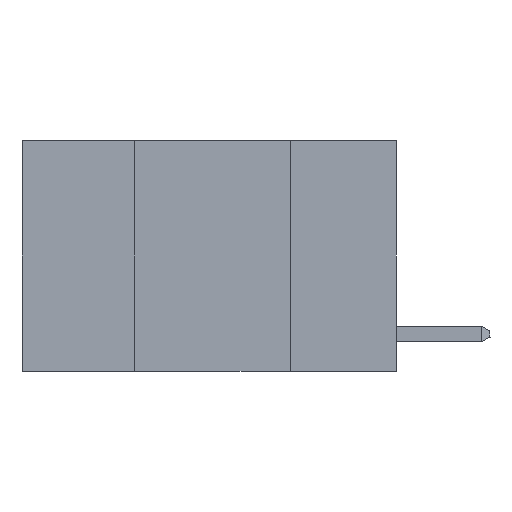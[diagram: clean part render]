
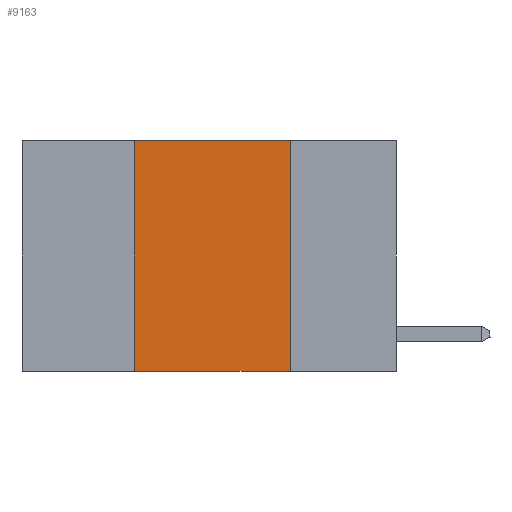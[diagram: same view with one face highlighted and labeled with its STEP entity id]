
A CAD part, left-side view. The second image highlights one B-rep face of the part: STEP entity #9163.
In plain terms, the highlighted planar face has unit normal (-1, 0, 0).
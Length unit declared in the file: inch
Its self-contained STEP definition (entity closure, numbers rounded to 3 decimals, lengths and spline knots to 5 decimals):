
#3 = ORIENTED_EDGE ( 'NONE', *, *, #9107, .F. ) ;
#233 = VECTOR ( 'NONE', #1247, 39.37008 ) ;
#325 = VERTEX_POINT ( 'NONE', #587 ) ;
#587 = CARTESIAN_POINT ( 'NONE',  ( 0., 0.42, 0. ) ) ;
#1243 = EDGE_CURVE ( 'NONE', #5253, #9090, #6904, .T. ) ;
#1247 = DIRECTION ( 'NONE',  ( 0., 0., 1. ) ) ;
#1419 = DIRECTION ( 'NONE',  ( 0., 0., -1. ) ) ;
#1798 = CARTESIAN_POINT ( 'NONE',  ( 0., 0.6, -0.37 ) ) ;
#1821 = VECTOR ( 'NONE', #6921, 39.37008 ) ;
#1911 = PLANE ( 'NONE',  #3195 ) ;
#1963 = ORIENTED_EDGE ( 'NONE', *, *, #5374, .F. ) ;
#2168 = ORIENTED_EDGE ( 'NONE', *, *, #5961, .F. ) ;
#2296 = DIRECTION ( 'NONE',  ( 1., 0., 0. ) ) ;
#2796 = VECTOR ( 'NONE', #9141, 39.37008 ) ;
#3195 = AXIS2_PLACEMENT_3D ( 'NONE', #8995, #2296, #8478 ) ;
#3243 = VECTOR ( 'NONE', #1419, 39.37008 ) ;
#3391 = CARTESIAN_POINT ( 'NONE',  ( 0., 0.6, 0. ) ) ;
#4456 = CARTESIAN_POINT ( 'NONE',  ( 0., 0.17, -0.37 ) ) ;
#4504 = VERTEX_POINT ( 'NONE', #6407 ) ;
#4969 = ORIENTED_EDGE ( 'NONE', *, *, #1243, .T. ) ;
#5253 = VERTEX_POINT ( 'NONE', #7615 ) ;
#5374 = EDGE_CURVE ( 'NONE', #325, #4504, #8587, .T. ) ;
#5636 = FACE_OUTER_BOUND ( 'NONE', #9394, .T. ) ;
#5739 = LINE ( 'NONE', #7501, #233 ) ;
#5960 = CARTESIAN_POINT ( 'NONE',  ( 0., 0.17, 0. ) ) ;
#5961 = EDGE_CURVE ( 'NONE', #4504, #9090, #8226, .T. ) ;
#6407 = CARTESIAN_POINT ( 'NONE',  ( 0., 0.17, 0. ) ) ;
#6904 = LINE ( 'NONE', #1798, #2796 ) ;
#6921 = DIRECTION ( 'NONE',  ( 0., -1., 0. ) ) ;
#7501 = CARTESIAN_POINT ( 'NONE',  ( 0., 0.42, 0. ) ) ;
#7615 = CARTESIAN_POINT ( 'NONE',  ( 0., 0.42, -0.37 ) ) ;
#8226 = LINE ( 'NONE', #5960, #3243 ) ;
#8478 = DIRECTION ( 'NONE',  ( 0., 0., -1. ) ) ;
#8587 = LINE ( 'NONE', #3391, #1821 ) ;
#8995 = CARTESIAN_POINT ( 'NONE',  ( 0., 0.6, 0. ) ) ;
#9090 = VERTEX_POINT ( 'NONE', #4456 ) ;
#9107 = EDGE_CURVE ( 'NONE', #5253, #325, #5739, .T. ) ;
#9141 = DIRECTION ( 'NONE',  ( 0., -1., 0. ) ) ;
#9163 = ADVANCED_FACE ( 'NONE', ( #5636 ), #1911, .F. ) ;
#9394 = EDGE_LOOP ( 'NONE', ( #2168, #1963, #3, #4969 ) ) ;
